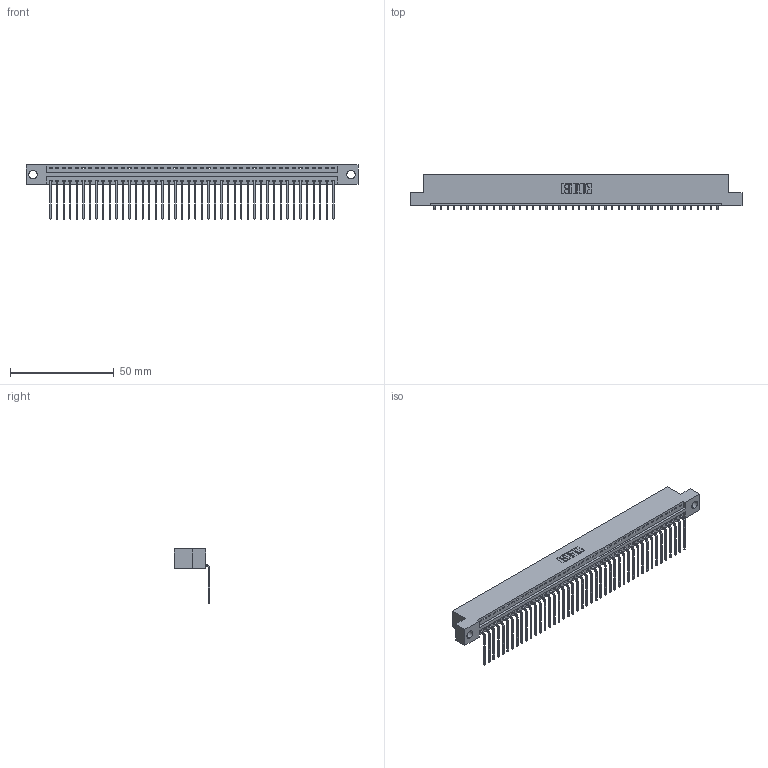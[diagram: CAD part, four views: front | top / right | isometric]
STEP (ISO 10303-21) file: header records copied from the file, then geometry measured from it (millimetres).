
FILE_DESCRIPTION (( 'STEP AP203' ), '1' );
FILE_NAME ('346-044-559-104.STEP', '2018-08-25T02:51:02', ( '' ), ( '' ), 'SwSTEP 2.0', 'SolidWorks 2016', '' );
FILE_SCHEMA (( 'CONFIG_CONTROL_DESIGN' ));
Length unit declared in the file: inch
Products named in the file (3): 346 Part_Flush Mounting Lugs - 0.156 Dia-TH; 345-292-001_558 559 Tail - 1; 346-044-559-104
Assembly tree (45 placements, depth 2):
  346-044-559-104
    346 Part_Flush Mounting Lugs - 0.156 Dia-TH
    345-292-001_558 559 Tail - 1  x44
Bounding box: 160.27 x 17.08 x 26.16 mm (x, y, z)
Volume: 15414.3 mm3; surface area: 19967 mm2
Topology: 45 solids, 45 shells, 2762 faces, 8337 edges, 5498 vertices
Faces by surface type: plane 1924, cylinder 838
Entity records: 27125 total; most frequent: CARTESIAN_POINT 4656, ORIENTED_EDGE 4634, DIRECTION 4105, EDGE_CURVE 2317, LINE 2009, VECTOR 2009, VERTEX_POINT 1542, AXIS2_PLACEMENT_3D 1048
